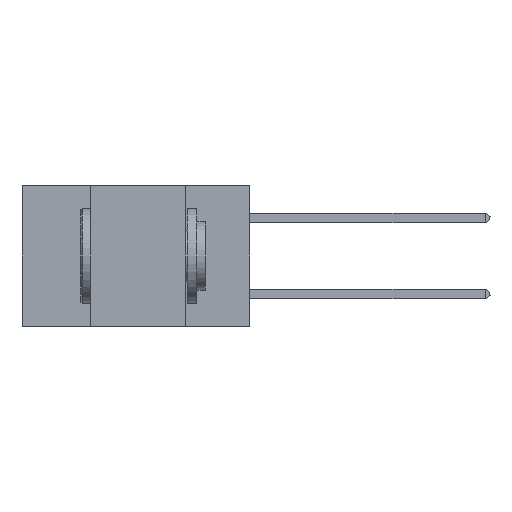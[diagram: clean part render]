
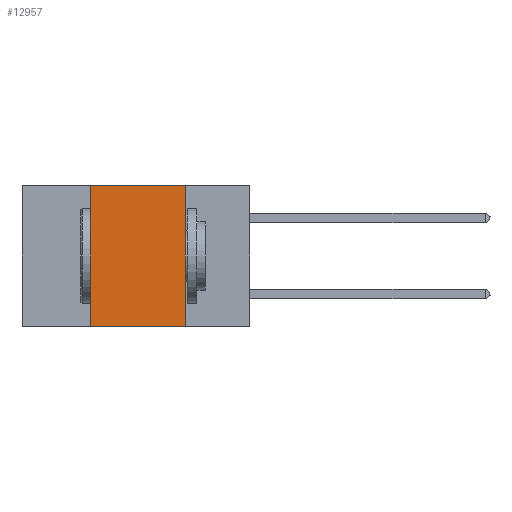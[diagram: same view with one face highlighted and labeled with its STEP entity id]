
A CAD part, left-side view. The second image highlights one B-rep face of the part: STEP entity #12957.
In plain terms, the highlighted planar face has unit normal (-1, 0, 0).
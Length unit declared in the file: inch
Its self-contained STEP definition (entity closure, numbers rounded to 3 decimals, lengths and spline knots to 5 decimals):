
#163 = VECTOR ( 'NONE', #30825, 39.37008 ) ;
#449 = VERTEX_POINT ( 'NONE', #26163 ) ;
#3094 = ORIENTED_EDGE ( 'NONE', *, *, #8001, .T. ) ;
#6040 = ORIENTED_EDGE ( 'NONE', *, *, #35181, .F. ) ;
#8001 = EDGE_CURVE ( 'NONE', #23990, #8710, #10910, .T. ) ;
#8710 = VERTEX_POINT ( 'NONE', #20097 ) ;
#10910 = LINE ( 'NONE', #19384, #15759 ) ;
#11436 = VERTEX_POINT ( 'NONE', #20428 ) ;
#11525 = CARTESIAN_POINT ( 'NONE',  ( 0., 0.17, 0. ) ) ;
#11527 = PLANE ( 'NONE',  #25039 ) ;
#12673 = VECTOR ( 'NONE', #22803, 39.37008 ) ;
#12957 = ADVANCED_FACE ( 'NONE', ( #20595 ), #11527, .F. ) ;
#13817 = DIRECTION ( 'NONE',  ( 0., 0., -1. ) ) ;
#15759 = VECTOR ( 'NONE', #33125, 39.37008 ) ;
#16400 = CARTESIAN_POINT ( 'NONE',  ( 0., 0.42, 0. ) ) ;
#16516 = DIRECTION ( 'NONE',  ( 0., 0., 1. ) ) ;
#19384 = CARTESIAN_POINT ( 'NONE',  ( 0., 0.6, -0.37 ) ) ;
#20097 = CARTESIAN_POINT ( 'NONE',  ( 0., 0.17, -0.37 ) ) ;
#20204 = VECTOR ( 'NONE', #16516, 39.37008 ) ;
#20353 = ORIENTED_EDGE ( 'NONE', *, *, #33134, .F. ) ;
#20428 = CARTESIAN_POINT ( 'NONE',  ( 0., 0.42, 0. ) ) ;
#20595 = FACE_OUTER_BOUND ( 'NONE', #30720, .T. ) ;
#21142 = CARTESIAN_POINT ( 'NONE',  ( 0., 0.6, 0. ) ) ;
#22803 = DIRECTION ( 'NONE',  ( 0., 0., -1. ) ) ;
#23553 = EDGE_CURVE ( 'NONE', #11436, #449, #27047, .T. ) ;
#23990 = VERTEX_POINT ( 'NONE', #28835 ) ;
#25039 = AXIS2_PLACEMENT_3D ( 'NONE', #31312, #26650, #13817 ) ;
#26163 = CARTESIAN_POINT ( 'NONE',  ( 0., 0.17, 0. ) ) ;
#26650 = DIRECTION ( 'NONE',  ( 1., 0., 0. ) ) ;
#27047 = LINE ( 'NONE', #21142, #163 ) ;
#28835 = CARTESIAN_POINT ( 'NONE',  ( 0., 0.42, -0.37 ) ) ;
#30720 = EDGE_LOOP ( 'NONE', ( #6040, #31857, #20353, #3094 ) ) ;
#30825 = DIRECTION ( 'NONE',  ( 0., -1., 0. ) ) ;
#31312 = CARTESIAN_POINT ( 'NONE',  ( 0., 0.6, 0. ) ) ;
#31857 = ORIENTED_EDGE ( 'NONE', *, *, #23553, .F. ) ;
#32363 = LINE ( 'NONE', #11525, #12673 ) ;
#33125 = DIRECTION ( 'NONE',  ( 0., -1., 0. ) ) ;
#33134 = EDGE_CURVE ( 'NONE', #23990, #11436, #33661, .T. ) ;
#33661 = LINE ( 'NONE', #16400, #20204 ) ;
#35181 = EDGE_CURVE ( 'NONE', #449, #8710, #32363, .T. ) ;
